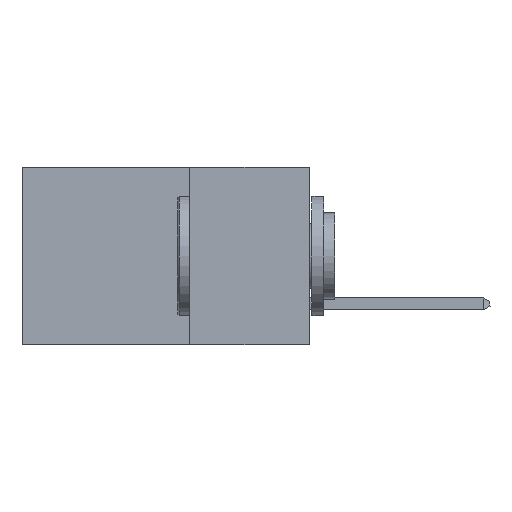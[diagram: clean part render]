
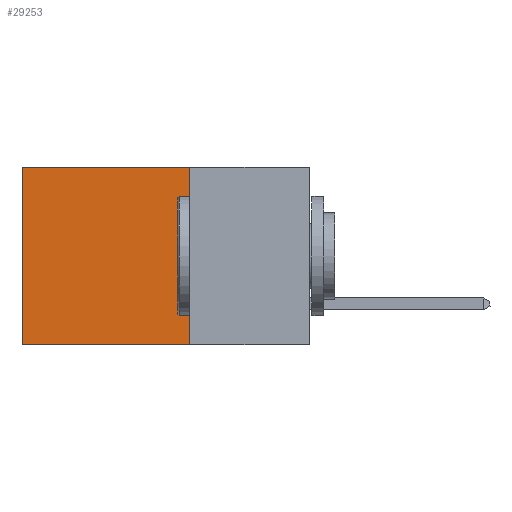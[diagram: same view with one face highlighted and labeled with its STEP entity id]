
A CAD part, left-side view. The second image highlights one B-rep face of the part: STEP entity #29253.
In plain terms, the highlighted planar face has unit normal (-1, 0, 0).
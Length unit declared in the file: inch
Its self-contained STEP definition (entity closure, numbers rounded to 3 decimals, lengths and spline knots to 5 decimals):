
#666 = CARTESIAN_POINT ( 'NONE',  ( 0.2875, 0.6, -0.37 ) ) ;
#956 = EDGE_CURVE ( 'NONE', #39347, #26891, #25801, .T. ) ;
#1447 = DIRECTION ( 'NONE',  ( 0., 0., -1. ) ) ;
#2297 = VECTOR ( 'NONE', #34863, 39.37008 ) ;
#3109 = EDGE_CURVE ( 'NONE', #38168, #39347, #20182, .T. ) ;
#3867 = VECTOR ( 'NONE', #1447, 39.37008 ) ;
#4669 = CARTESIAN_POINT ( 'NONE',  ( 0.2875, 0.25, 0. ) ) ;
#5151 = DIRECTION ( 'NONE',  ( 1., 0., 0. ) ) ;
#9314 = ORIENTED_EDGE ( 'NONE', *, *, #22008, .F. ) ;
#9688 = CARTESIAN_POINT ( 'NONE',  ( 0.2875, 0.25, 0. ) ) ;
#12180 = CARTESIAN_POINT ( 'NONE',  ( 0.2875, 0.25, 0. ) ) ;
#12192 = DIRECTION ( 'NONE',  ( 0., 0., -1. ) ) ;
#14018 = LINE ( 'NONE', #35078, #29778 ) ;
#17099 = FACE_OUTER_BOUND ( 'NONE', #33125, .T. ) ;
#20182 = LINE ( 'NONE', #9688, #2297 ) ;
#22008 = EDGE_CURVE ( 'NONE', #38168, #37975, #35497, .T. ) ;
#24808 = VECTOR ( 'NONE', #12192, 39.37008 ) ;
#25801 = LINE ( 'NONE', #34175, #24808 ) ;
#26891 = VERTEX_POINT ( 'NONE', #666 ) ;
#27361 = DIRECTION ( 'NONE',  ( 0., 0., -1. ) ) ;
#27711 = ORIENTED_EDGE ( 'NONE', *, *, #956, .T. ) ;
#29046 = ORIENTED_EDGE ( 'NONE', *, *, #31382, .F. ) ;
#29253 = ADVANCED_FACE ( 'NONE', ( #17099 ), #39606, .F. ) ;
#29724 = AXIS2_PLACEMENT_3D ( 'NONE', #39742, #5151, #27361 ) ;
#29778 = VECTOR ( 'NONE', #38231, 39.37008 ) ;
#31021 = ORIENTED_EDGE ( 'NONE', *, *, #3109, .T. ) ;
#31360 = CARTESIAN_POINT ( 'NONE',  ( 0.2875, 0.6, 0. ) ) ;
#31382 = EDGE_CURVE ( 'NONE', #37975, #26891, #14018, .T. ) ;
#33125 = EDGE_LOOP ( 'NONE', ( #27711, #29046, #9314, #31021 ) ) ;
#34175 = CARTESIAN_POINT ( 'NONE',  ( 0.2875, 0.6, 0. ) ) ;
#34863 = DIRECTION ( 'NONE',  ( 0., 1., 0. ) ) ;
#35078 = CARTESIAN_POINT ( 'NONE',  ( 0.2875, 0.25, -0.37 ) ) ;
#35497 = LINE ( 'NONE', #4669, #3867 ) ;
#36387 = CARTESIAN_POINT ( 'NONE',  ( 0.2875, 0.25, -0.37 ) ) ;
#37975 = VERTEX_POINT ( 'NONE', #36387 ) ;
#38168 = VERTEX_POINT ( 'NONE', #12180 ) ;
#38231 = DIRECTION ( 'NONE',  ( 0., 1., 0. ) ) ;
#39347 = VERTEX_POINT ( 'NONE', #31360 ) ;
#39606 = PLANE ( 'NONE',  #29724 ) ;
#39742 = CARTESIAN_POINT ( 'NONE',  ( 0.2875, 0.25, 0. ) ) ;
